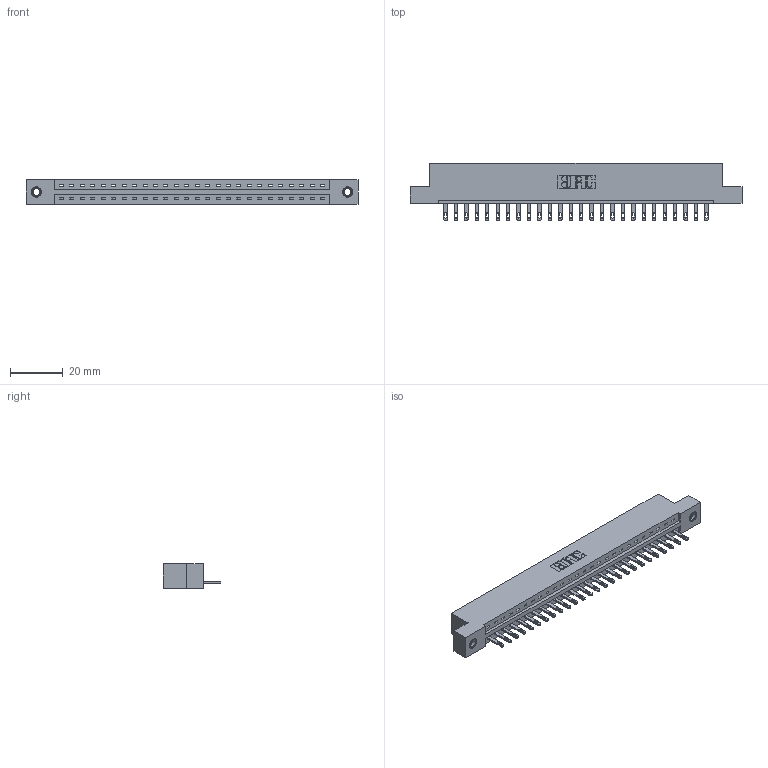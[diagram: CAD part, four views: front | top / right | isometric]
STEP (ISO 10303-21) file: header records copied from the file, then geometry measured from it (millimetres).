
FILE_DESCRIPTION (( 'STEP AP203' ), '1' );
FILE_NAME ('337-026-500-107.STEP', '2019-09-30T18:10:20', ( '' ), ( '' ), 'SwSTEP 2.0', 'SolidWorks 2016', '' );
FILE_SCHEMA (( 'CONFIG_CONTROL_DESIGN' ));
Length unit declared in the file: inch
Products named in the file (4): 337 Part_Flush Mounting Lugs - 0.156 Dia-TI; 345-292-001_345-293-100; 345-250-001_345-250-005-103; 337-026-500-107
Assembly tree (29 placements, depth 2):
  337-026-500-107
    337 Part_Flush Mounting Lugs - 0.156 Dia-TI
    345-292-001_345-293-100  x26
    345-250-001_345-250-005-103  x2
Bounding box: 126.03 x 21.85 x 9.4 mm (x, y, z)
Volume: 12901.6 mm3; surface area: 13344.8 mm2
Topology: 29 solids, 29 shells, 1682 faces, 5127 edges, 3410 vertices
Faces by surface type: plane 1142, cylinder 524, cone 12, torus 4
Entity records: 22512 total; most frequent: CARTESIAN_POINT 3899, ORIENTED_EDGE 3854, DIRECTION 3349, EDGE_CURVE 1927, VECTOR 1775, LINE 1775, VERTEX_POINT 1280, AXIS2_PLACEMENT_3D 787
